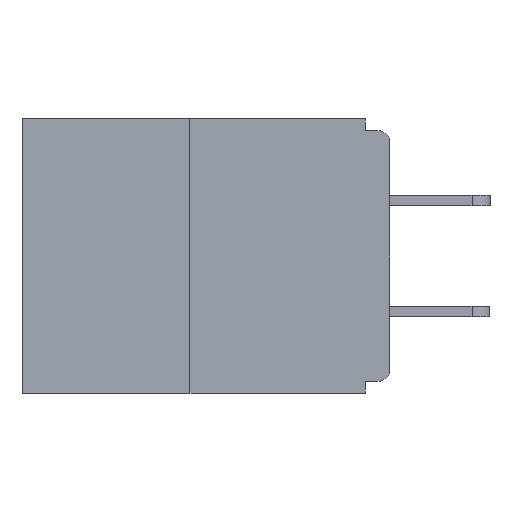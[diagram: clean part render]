
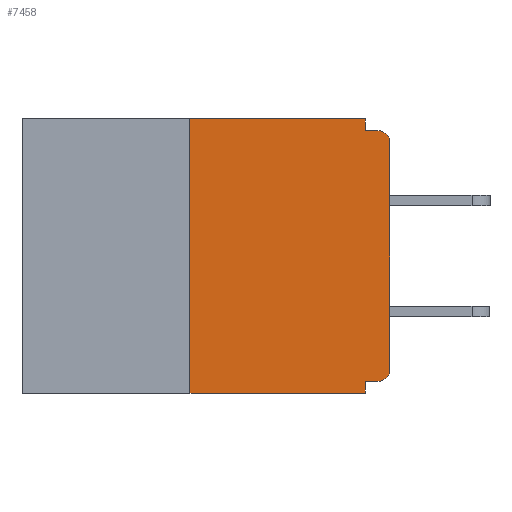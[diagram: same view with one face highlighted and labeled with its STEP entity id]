
A CAD part, left-side view. The second image highlights one B-rep face of the part: STEP entity #7458.
In plain terms, the highlighted planar face has unit normal (-1, 0, 0).
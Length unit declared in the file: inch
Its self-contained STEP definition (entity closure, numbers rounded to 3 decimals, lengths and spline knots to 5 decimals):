
#1 = DIRECTION ( 'NONE',  ( 0., -1., 0. ) ) ;
#141 = DIRECTION ( 'NONE',  ( -1., 0., 0. ) ) ;
#197 = DIRECTION ( 'NONE',  ( 0., 0., -1. ) ) ;
#303 = DIRECTION ( 'NONE',  ( 0., -1., 0. ) ) ;
#433 = PLANE ( 'NONE',  #11146 ) ;
#608 = VERTEX_POINT ( 'NONE', #3296 ) ;
#953 = EDGE_CURVE ( 'NONE', #7429, #2787, #4334, .T. ) ;
#1489 = DIRECTION ( 'NONE',  ( 0., 0., 1. ) ) ;
#1824 = VECTOR ( 'NONE', #1, 39.37008 ) ;
#2481 = CARTESIAN_POINT ( 'NONE',  ( 0., 0., -0.313 ) ) ;
#2550 = LINE ( 'NONE', #11412, #8201 ) ;
#2629 = EDGE_CURVE ( 'NONE', #4691, #608, #13282, .T. ) ;
#2681 = VECTOR ( 'NONE', #8614, 39.37008 ) ;
#2787 = VERTEX_POINT ( 'NONE', #8353 ) ;
#3296 = CARTESIAN_POINT ( 'NONE',  ( 0., 0.031, -0.343 ) ) ;
#3383 = AXIS2_PLACEMENT_3D ( 'NONE', #13745, #141, #197 ) ;
#3388 = CARTESIAN_POINT ( 'NONE',  ( 0., 0.46, -0.343 ) ) ;
#3543 = CIRCLE ( 'NONE', #3383, 0.015 ) ;
#3573 = DIRECTION ( 'NONE',  ( 0., 0., -1. ) ) ;
#3695 = EDGE_CURVE ( 'NONE', #6589, #8909, #6536, .T. ) ;
#4240 = VECTOR ( 'NONE', #11689, 39.37008 ) ;
#4334 = LINE ( 'NONE', #8246, #5226 ) ;
#4435 = ORIENTED_EDGE ( 'NONE', *, *, #8979, .T. ) ;
#4607 = DIRECTION ( 'NONE',  ( 0., -1., 0. ) ) ;
#4691 = VERTEX_POINT ( 'NONE', #9282 ) ;
#4798 = LINE ( 'NONE', #5008, #4240 ) ;
#4952 = CARTESIAN_POINT ( 'NONE',  ( 0., 0.46, 0. ) ) ;
#4975 = LINE ( 'NONE', #5782, #2681 ) ;
#5008 = CARTESIAN_POINT ( 'NONE',  ( 0., 0.031, 0. ) ) ;
#5226 = VECTOR ( 'NONE', #1489, 39.37008 ) ;
#5306 = VECTOR ( 'NONE', #303, 39.37008 ) ;
#5397 = FACE_OUTER_BOUND ( 'NONE', #9922, .T. ) ;
#5775 = ORIENTED_EDGE ( 'NONE', *, *, #14504, .T. ) ;
#5782 = CARTESIAN_POINT ( 'NONE',  ( 0., 0., -0.328 ) ) ;
#6092 = DIRECTION ( 'NONE',  ( 0., 0., -1. ) ) ;
#6179 = EDGE_CURVE ( 'NONE', #7291, #8522, #9159, .T. ) ;
#6463 = ORIENTED_EDGE ( 'NONE', *, *, #8821, .F. ) ;
#6536 = LINE ( 'NONE', #11693, #5306 ) ;
#6589 = VERTEX_POINT ( 'NONE', #11474 ) ;
#6895 = DIRECTION ( 'NONE',  ( 0., 0., -1. ) ) ;
#7291 = VERTEX_POINT ( 'NONE', #8850 ) ;
#7429 = VERTEX_POINT ( 'NONE', #2481 ) ;
#7458 = ADVANCED_FACE ( 'NONE', ( #5397 ), #433, .F. ) ;
#7705 = ORIENTED_EDGE ( 'NONE', *, *, #14254, .F. ) ;
#7708 = VERTEX_POINT ( 'NONE', #7977 ) ;
#7797 = CARTESIAN_POINT ( 'NONE',  ( 0., 0.031, 0. ) ) ;
#7942 = CARTESIAN_POINT ( 'NONE',  ( 0., 0.015, -0.313 ) ) ;
#7977 = CARTESIAN_POINT ( 'NONE',  ( 0., 0.031, -0.328 ) ) ;
#8201 = VECTOR ( 'NONE', #6895, 39.37008 ) ;
#8246 = CARTESIAN_POINT ( 'NONE',  ( 0., 0., 0. ) ) ;
#8353 = CARTESIAN_POINT ( 'NONE',  ( 0., 0., -0.03 ) ) ;
#8522 = VERTEX_POINT ( 'NONE', #14485 ) ;
#8614 = DIRECTION ( 'NONE',  ( 0., 1., 0. ) ) ;
#8821 = EDGE_CURVE ( 'NONE', #13669, #7708, #4975, .T. ) ;
#8850 = CARTESIAN_POINT ( 'NONE',  ( 0., 0.031, -0.015 ) ) ;
#8909 = VERTEX_POINT ( 'NONE', #7797 ) ;
#8979 = EDGE_CURVE ( 'NONE', #2787, #8522, #3543, .T. ) ;
#9159 = LINE ( 'NONE', #12352, #10374 ) ;
#9282 = CARTESIAN_POINT ( 'NONE',  ( 0., 0.25, -0.343 ) ) ;
#9922 = EDGE_LOOP ( 'NONE', ( #13482, #7705, #10051, #14268, #6463, #5775, #9941, #4435, #14259, #10516 ) ) ;
#9941 = ORIENTED_EDGE ( 'NONE', *, *, #953, .T. ) ;
#10051 = ORIENTED_EDGE ( 'NONE', *, *, #2629, .T. ) ;
#10196 = AXIS2_PLACEMENT_3D ( 'NONE', #7942, #13642, #3573 ) ;
#10374 = VECTOR ( 'NONE', #4607, 39.37008 ) ;
#10516 = ORIENTED_EDGE ( 'NONE', *, *, #10996, .F. ) ;
#10872 = VECTOR ( 'NONE', #11279, 39.37008 ) ;
#10996 = EDGE_CURVE ( 'NONE', #8909, #7291, #4798, .T. ) ;
#11146 = AXIS2_PLACEMENT_3D ( 'NONE', #4952, #11628, #6092 ) ;
#11279 = DIRECTION ( 'NONE',  ( 0., 0., 1. ) ) ;
#11412 = CARTESIAN_POINT ( 'NONE',  ( 0., 0.031, -0.343 ) ) ;
#11474 = CARTESIAN_POINT ( 'NONE',  ( 0., 0.25, 0. ) ) ;
#11628 = DIRECTION ( 'NONE',  ( 1., 0., 0. ) ) ;
#11689 = DIRECTION ( 'NONE',  ( 0., 0., -1. ) ) ;
#11693 = CARTESIAN_POINT ( 'NONE',  ( 0., 0.46, 0. ) ) ;
#12084 = CIRCLE ( 'NONE', #10196, 0.015 ) ;
#12352 = CARTESIAN_POINT ( 'NONE',  ( 0., 0., -0.015 ) ) ;
#12468 = CARTESIAN_POINT ( 'NONE',  ( 0., 0.25, 0. ) ) ;
#13282 = LINE ( 'NONE', #3388, #1824 ) ;
#13482 = ORIENTED_EDGE ( 'NONE', *, *, #3695, .F. ) ;
#13637 = CARTESIAN_POINT ( 'NONE',  ( 0., 0.015, -0.328 ) ) ;
#13642 = DIRECTION ( 'NONE',  ( -1., 0., 0. ) ) ;
#13669 = VERTEX_POINT ( 'NONE', #13637 ) ;
#13745 = CARTESIAN_POINT ( 'NONE',  ( 0., 0.015, -0.03 ) ) ;
#14032 = LINE ( 'NONE', #12468, #10872 ) ;
#14254 = EDGE_CURVE ( 'NONE', #4691, #6589, #14032, .T. ) ;
#14259 = ORIENTED_EDGE ( 'NONE', *, *, #6179, .F. ) ;
#14268 = ORIENTED_EDGE ( 'NONE', *, *, #14569, .F. ) ;
#14485 = CARTESIAN_POINT ( 'NONE',  ( 0., 0.015, -0.015 ) ) ;
#14504 = EDGE_CURVE ( 'NONE', #13669, #7429, #12084, .T. ) ;
#14569 = EDGE_CURVE ( 'NONE', #7708, #608, #2550, .T. ) ;
